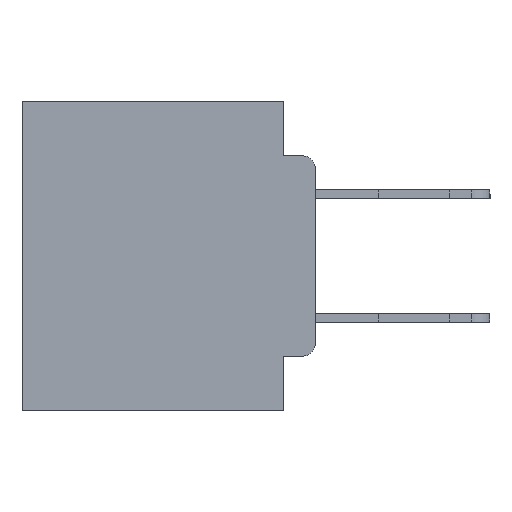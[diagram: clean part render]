
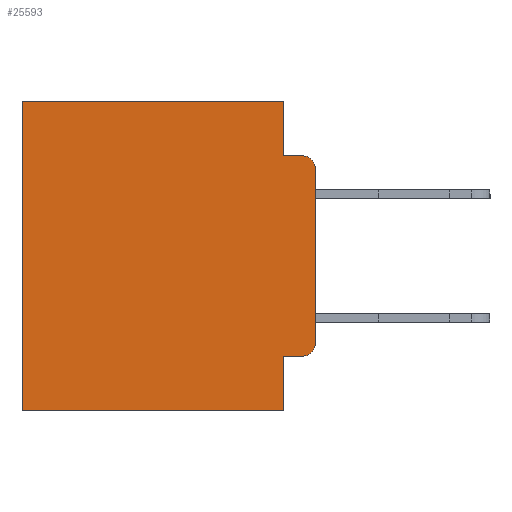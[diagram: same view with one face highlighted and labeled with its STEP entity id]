
A CAD part, left-side view. The second image highlights one B-rep face of the part: STEP entity #25593.
In plain terms, the highlighted planar face has unit normal (-1, 0, 0).
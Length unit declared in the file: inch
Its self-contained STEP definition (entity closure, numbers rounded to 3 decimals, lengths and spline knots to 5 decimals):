
#598 = ORIENTED_EDGE ( 'NONE', *, *, #11427, .F. ) ;
#612 = CARTESIAN_POINT ( 'NONE',  ( 0.298, 0.051, 0. ) ) ;
#1043 = DIRECTION ( 'NONE',  ( 0., 0., -1. ) ) ;
#1224 = VECTOR ( 'NONE', #26002, 39.37008 ) ;
#1293 = LINE ( 'NONE', #4156, #7470 ) ;
#1510 = EDGE_CURVE ( 'NONE', #8189, #9868, #9987, .T. ) ;
#1635 = ORIENTED_EDGE ( 'NONE', *, *, #9948, .T. ) ;
#1726 = VECTOR ( 'NONE', #21933, 39.37008 ) ;
#1967 = LINE ( 'NONE', #17219, #1224 ) ;
#2344 = CARTESIAN_POINT ( 'NONE',  ( 0.298, 0., -0.5 ) ) ;
#2469 = LINE ( 'NONE', #26226, #1726 ) ;
#2512 = ORIENTED_EDGE ( 'NONE', *, *, #1510, .F. ) ;
#2704 = DIRECTION ( 'NONE',  ( 0., 1., 0. ) ) ;
#3059 = VECTOR ( 'NONE', #7832, 39.37008 ) ;
#3079 = ORIENTED_EDGE ( 'NONE', *, *, #21614, .T. ) ;
#3706 = CARTESIAN_POINT ( 'NONE',  ( 0.298, 0.051, -0.0885 ) ) ;
#3825 = EDGE_CURVE ( 'NONE', #4265, #15071, #26803, .T. ) ;
#4156 = CARTESIAN_POINT ( 'NONE',  ( 0.298, 0.051, 0. ) ) ;
#4171 = CARTESIAN_POINT ( 'NONE',  ( 0.298, 0.051, -0.4115 ) ) ;
#4265 = VERTEX_POINT ( 'NONE', #4171 ) ;
#4543 = ORIENTED_EDGE ( 'NONE', *, *, #3825, .T. ) ;
#4694 = AXIS2_PLACEMENT_3D ( 'NONE', #10229, #25688, #12451 ) ;
#5665 = DIRECTION ( 'NONE',  ( 0., 0., -1. ) ) ;
#5821 = DIRECTION ( 'NONE',  ( 0., 1., 0. ) ) ;
#5929 = CARTESIAN_POINT ( 'NONE',  ( 0.298, 0., -0.3915 ) ) ;
#6910 = ORIENTED_EDGE ( 'NONE', *, *, #11760, .F. ) ;
#6935 = LINE ( 'NONE', #7942, #12172 ) ;
#7470 = VECTOR ( 'NONE', #26485, 39.37008 ) ;
#7493 = VERTEX_POINT ( 'NONE', #17982 ) ;
#7611 = CARTESIAN_POINT ( 'NONE',  ( 0.298, 0., 0. ) ) ;
#7832 = DIRECTION ( 'NONE',  ( 0., -1., 0. ) ) ;
#7942 = CARTESIAN_POINT ( 'NONE',  ( 0.298, 0., 0. ) ) ;
#8189 = VERTEX_POINT ( 'NONE', #24850 ) ;
#9022 = CIRCLE ( 'NONE', #10017, 0.02 ) ;
#9176 = CARTESIAN_POINT ( 'NONE',  ( 0.298, 0., -0.1085 ) ) ;
#9217 = LINE ( 'NONE', #612, #21067 ) ;
#9261 = ORIENTED_EDGE ( 'NONE', *, *, #9813, .T. ) ;
#9676 = CIRCLE ( 'NONE', #4694, 0.02 ) ;
#9813 = EDGE_CURVE ( 'NONE', #25885, #21881, #24302, .T. ) ;
#9868 = VERTEX_POINT ( 'NONE', #27231 ) ;
#9948 = EDGE_CURVE ( 'NONE', #15071, #28081, #9022, .T. ) ;
#9987 = LINE ( 'NONE', #2344, #26241 ) ;
#10017 = AXIS2_PLACEMENT_3D ( 'NONE', #21921, #22245, #22263 ) ;
#10229 = CARTESIAN_POINT ( 'NONE',  ( 0.298, 0.02, -0.1085 ) ) ;
#10485 = FACE_OUTER_BOUND ( 'NONE', #26459, .T. ) ;
#11427 = EDGE_CURVE ( 'NONE', #4265, #8189, #9217, .T. ) ;
#11711 = CARTESIAN_POINT ( 'NONE',  ( 0.298, 0.473, 0. ) ) ;
#11760 = EDGE_CURVE ( 'NONE', #25885, #19247, #1293, .T. ) ;
#12172 = VECTOR ( 'NONE', #1043, 39.37008 ) ;
#12451 = DIRECTION ( 'NONE',  ( 0., 0., -1. ) ) ;
#13053 = CARTESIAN_POINT ( 'NONE',  ( 0.298, 0.02, -0.4115 ) ) ;
#13437 = ORIENTED_EDGE ( 'NONE', *, *, #20883, .T. ) ;
#15071 = VERTEX_POINT ( 'NONE', #13053 ) ;
#16037 = ORIENTED_EDGE ( 'NONE', *, *, #18083, .F. ) ;
#16355 = ORIENTED_EDGE ( 'NONE', *, *, #26208, .F. ) ;
#16472 = DIRECTION ( 'NONE',  ( 0., 0., -1. ) ) ;
#16814 = PLANE ( 'NONE',  #22766 ) ;
#17219 = CARTESIAN_POINT ( 'NONE',  ( 0.298, 0.051, -0.0885 ) ) ;
#17697 = VERTEX_POINT ( 'NONE', #9176 ) ;
#17982 = CARTESIAN_POINT ( 'NONE',  ( 0.298, 0.02, -0.0885 ) ) ;
#18083 = EDGE_CURVE ( 'NONE', #19247, #7493, #1967, .T. ) ;
#18438 = VECTOR ( 'NONE', #5821, 39.37008 ) ;
#19048 = DIRECTION ( 'NONE',  ( 1., 0., 0. ) ) ;
#19247 = VERTEX_POINT ( 'NONE', #3706 ) ;
#20883 = EDGE_CURVE ( 'NONE', #17697, #7493, #9676, .T. ) ;
#21067 = VECTOR ( 'NONE', #16472, 39.37008 ) ;
#21614 = EDGE_CURVE ( 'NONE', #21881, #9868, #2469, .T. ) ;
#21881 = VERTEX_POINT ( 'NONE', #11711 ) ;
#21921 = CARTESIAN_POINT ( 'NONE',  ( 0.298, 0.02, -0.3915 ) ) ;
#21933 = DIRECTION ( 'NONE',  ( 0., 0., -1. ) ) ;
#22245 = DIRECTION ( 'NONE',  ( -1., 0., 0. ) ) ;
#22263 = DIRECTION ( 'NONE',  ( 0., 0., -1. ) ) ;
#22766 = AXIS2_PLACEMENT_3D ( 'NONE', #25586, #19048, #5665 ) ;
#24302 = LINE ( 'NONE', #7611, #18438 ) ;
#24850 = CARTESIAN_POINT ( 'NONE',  ( 0.298, 0.051, -0.5 ) ) ;
#25517 = CARTESIAN_POINT ( 'NONE',  ( 0.298, 0.051, -0.4115 ) ) ;
#25586 = CARTESIAN_POINT ( 'NONE',  ( 0.298, 0., 0. ) ) ;
#25593 = ADVANCED_FACE ( 'NONE', ( #10485 ), #16814, .F. ) ;
#25688 = DIRECTION ( 'NONE',  ( -1., 0., 0. ) ) ;
#25885 = VERTEX_POINT ( 'NONE', #26536 ) ;
#26002 = DIRECTION ( 'NONE',  ( 0., -1., 0. ) ) ;
#26208 = EDGE_CURVE ( 'NONE', #17697, #28081, #6935, .T. ) ;
#26226 = CARTESIAN_POINT ( 'NONE',  ( 0.298, 0.473, 0. ) ) ;
#26241 = VECTOR ( 'NONE', #2704, 39.37008 ) ;
#26459 = EDGE_LOOP ( 'NONE', ( #16355, #13437, #16037, #6910, #9261, #3079, #2512, #598, #4543, #1635 ) ) ;
#26485 = DIRECTION ( 'NONE',  ( 0., 0., -1. ) ) ;
#26536 = CARTESIAN_POINT ( 'NONE',  ( 0.298, 0.051, 0. ) ) ;
#26803 = LINE ( 'NONE', #25517, #3059 ) ;
#27231 = CARTESIAN_POINT ( 'NONE',  ( 0.298, 0.473, -0.5 ) ) ;
#28081 = VERTEX_POINT ( 'NONE', #5929 ) ;
